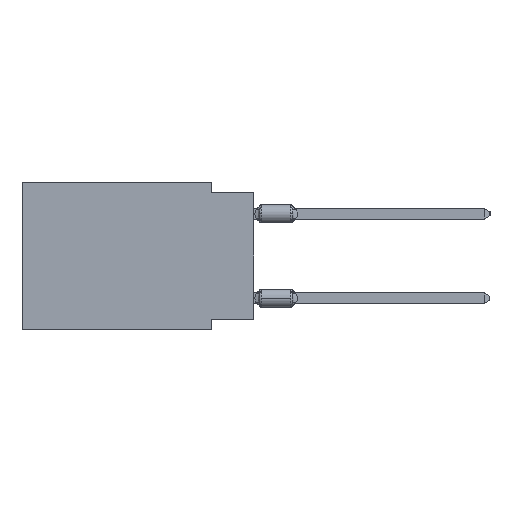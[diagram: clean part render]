
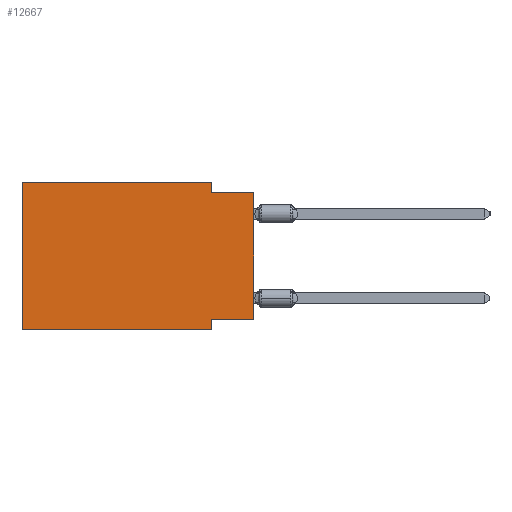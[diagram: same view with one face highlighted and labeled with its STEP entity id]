
A CAD part, left-side view. The second image highlights one B-rep face of the part: STEP entity #12667.
In plain terms, the highlighted planar face has unit normal (-1, 0, 0).
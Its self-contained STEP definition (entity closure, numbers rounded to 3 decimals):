
#221 = CARTESIAN_POINT ( 'NONE',  ( 0., 2.54, -0.635 ) ) ;
#392 = CARTESIAN_POINT ( 'NONE',  ( 0., 2.54, 0. ) ) ;
#572 = CARTESIAN_POINT ( 'NONE',  ( 0., 13.97, 0. ) ) ;
#1076 = ORIENTED_EDGE ( 'NONE', *, *, #3671, .F. ) ;
#1460 = CARTESIAN_POINT ( 'NONE',  ( 0., 13.97, -8.89 ) ) ;
#1483 = LINE ( 'NONE', #5003, #5651 ) ;
#2457 = DIRECTION ( 'NONE',  ( 1., 0., 0. ) ) ;
#2774 = VERTEX_POINT ( 'NONE', #23437 ) ;
#3126 = EDGE_LOOP ( 'NONE', ( #13674, #9344, #25806, #1076, #19978, #25349, #11741, #25155 ) ) ;
#3173 = DIRECTION ( 'NONE',  ( 0., 0., 1. ) ) ;
#3671 = EDGE_CURVE ( 'NONE', #14408, #8365, #21409, .T. ) ;
#3874 = LINE ( 'NONE', #18077, #5289 ) ;
#3890 = CARTESIAN_POINT ( 'NONE',  ( 0., 13.97, 0. ) ) ;
#4445 = PLANE ( 'NONE',  #25506 ) ;
#4635 = CARTESIAN_POINT ( 'NONE',  ( 0., 0., -0.635 ) ) ;
#4868 = DIRECTION ( 'NONE',  ( 0., 0., -1. ) ) ;
#5003 = CARTESIAN_POINT ( 'NONE',  ( 0., 2.54, 0. ) ) ;
#5289 = VECTOR ( 'NONE', #7999, 1000. ) ;
#5413 = CARTESIAN_POINT ( 'NONE',  ( 0., 0., -8.255 ) ) ;
#5651 = VECTOR ( 'NONE', #4868, 1000. ) ;
#6068 = DIRECTION ( 'NONE',  ( 0., 0., 1. ) ) ;
#6188 = EDGE_CURVE ( 'NONE', #2774, #19093, #17459, .T. ) ;
#6271 = VERTEX_POINT ( 'NONE', #221 ) ;
#7441 = CARTESIAN_POINT ( 'NONE',  ( 0., 2.54, -8.89 ) ) ;
#7999 = DIRECTION ( 'NONE',  ( 0., -1., 0. ) ) ;
#8365 = VERTEX_POINT ( 'NONE', #392 ) ;
#8427 = FACE_OUTER_BOUND ( 'NONE', #3126, .T. ) ;
#8542 = EDGE_CURVE ( 'NONE', #6271, #23362, #14730, .T. ) ;
#8785 = EDGE_CURVE ( 'NONE', #2774, #23362, #18143, .T. ) ;
#9344 = ORIENTED_EDGE ( 'NONE', *, *, #8542, .F. ) ;
#9943 = VERTEX_POINT ( 'NONE', #20890 ) ;
#10064 = EDGE_CURVE ( 'NONE', #23620, #9943, #3874, .T. ) ;
#10561 = EDGE_CURVE ( 'NONE', #19093, #9943, #23745, .T. ) ;
#11644 = DIRECTION ( 'NONE',  ( 0., 1., 0. ) ) ;
#11741 = ORIENTED_EDGE ( 'NONE', *, *, #10561, .F. ) ;
#12076 = DIRECTION ( 'NONE',  ( 0., 0., -1. ) ) ;
#12398 = DIRECTION ( 'NONE',  ( 0., 0., -1. ) ) ;
#12547 = CARTESIAN_POINT ( 'NONE',  ( 0., 13.97, 0. ) ) ;
#12667 = ADVANCED_FACE ( 'NONE', ( #8427 ), #4445, .F. ) ;
#12724 = DIRECTION ( 'NONE',  ( 0., -1., 0. ) ) ;
#13134 = CARTESIAN_POINT ( 'NONE',  ( 0., 13.97, 0. ) ) ;
#13674 = ORIENTED_EDGE ( 'NONE', *, *, #8785, .T. ) ;
#14043 = CARTESIAN_POINT ( 'NONE',  ( 0., 0., 0. ) ) ;
#14218 = VECTOR ( 'NONE', #12076, 1000. ) ;
#14408 = VERTEX_POINT ( 'NONE', #3890 ) ;
#14730 = LINE ( 'NONE', #4635, #17518 ) ;
#16602 = VECTOR ( 'NONE', #11644, 1000. ) ;
#17459 = LINE ( 'NONE', #5413, #16602 ) ;
#17518 = VECTOR ( 'NONE', #12724, 1000. ) ;
#18077 = CARTESIAN_POINT ( 'NONE',  ( 0., 13.97, -8.89 ) ) ;
#18143 = LINE ( 'NONE', #14043, #22204 ) ;
#18315 = CARTESIAN_POINT ( 'NONE',  ( 0., 0., -0.635 ) ) ;
#19093 = VERTEX_POINT ( 'NONE', #22916 ) ;
#19978 = ORIENTED_EDGE ( 'NONE', *, *, #25444, .F. ) ;
#20875 = EDGE_CURVE ( 'NONE', #8365, #6271, #1483, .T. ) ;
#20890 = CARTESIAN_POINT ( 'NONE',  ( 0., 2.54, -8.89 ) ) ;
#21409 = LINE ( 'NONE', #572, #22649 ) ;
#22204 = VECTOR ( 'NONE', #6068, 1000. ) ;
#22649 = VECTOR ( 'NONE', #25097, 1000. ) ;
#22916 = CARTESIAN_POINT ( 'NONE',  ( 0., 2.54, -8.255 ) ) ;
#23362 = VERTEX_POINT ( 'NONE', #18315 ) ;
#23437 = CARTESIAN_POINT ( 'NONE',  ( 0., 0., -8.255 ) ) ;
#23620 = VERTEX_POINT ( 'NONE', #1460 ) ;
#23745 = LINE ( 'NONE', #7441, #14218 ) ;
#25047 = LINE ( 'NONE', #13134, #25263 ) ;
#25097 = DIRECTION ( 'NONE',  ( 0., -1., 0. ) ) ;
#25155 = ORIENTED_EDGE ( 'NONE', *, *, #6188, .F. ) ;
#25263 = VECTOR ( 'NONE', #3173, 1000. ) ;
#25349 = ORIENTED_EDGE ( 'NONE', *, *, #10064, .T. ) ;
#25444 = EDGE_CURVE ( 'NONE', #23620, #14408, #25047, .T. ) ;
#25506 = AXIS2_PLACEMENT_3D ( 'NONE', #12547, #2457, #12398 ) ;
#25806 = ORIENTED_EDGE ( 'NONE', *, *, #20875, .F. ) ;
